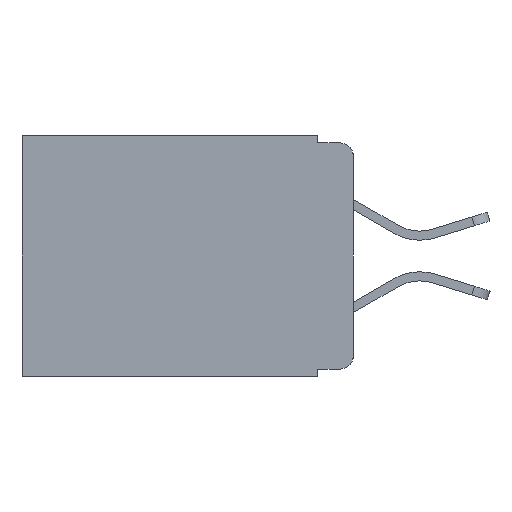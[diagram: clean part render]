
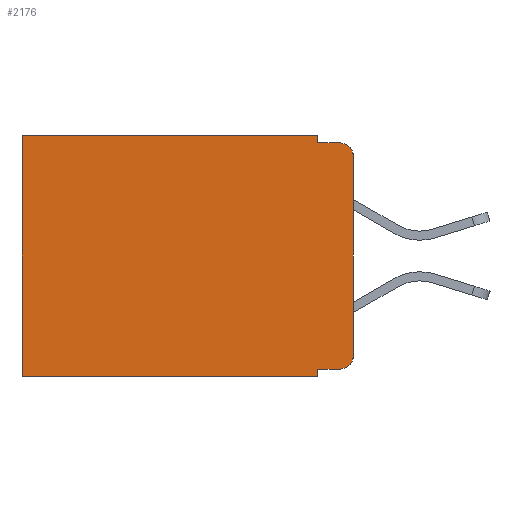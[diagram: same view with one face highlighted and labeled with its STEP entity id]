
A CAD part, left-side view. The second image highlights one B-rep face of the part: STEP entity #2176.
In plain terms, the highlighted planar face has unit normal (-1, 0, 0).
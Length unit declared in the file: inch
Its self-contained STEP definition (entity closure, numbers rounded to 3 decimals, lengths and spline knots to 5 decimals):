
#89 = DIRECTION ( 'NONE',  ( 0., 0., -1. ) ) ;
#152 = CARTESIAN_POINT ( 'NONE',  ( 0.298, 0., -0.313 ) ) ;
#309 = ORIENTED_EDGE ( 'NONE', *, *, #8397, .T. ) ;
#338 = DIRECTION ( 'NONE',  ( 0., 1., 0. ) ) ;
#526 = DIRECTION ( 'NONE',  ( 0., -1., 0. ) ) ;
#675 = VECTOR ( 'NONE', #7636, 39.37008 ) ;
#694 = CIRCLE ( 'NONE', #1011, 0.02 ) ;
#705 = CIRCLE ( 'NONE', #3646, 0.02 ) ;
#892 = ORIENTED_EDGE ( 'NONE', *, *, #9301, .F. ) ;
#983 = CARTESIAN_POINT ( 'NONE',  ( 0.298, 0., 0. ) ) ;
#1011 = AXIS2_PLACEMENT_3D ( 'NONE', #6147, #4822, #6840 ) ;
#1178 = ORIENTED_EDGE ( 'NONE', *, *, #4359, .T. ) ;
#1251 = CARTESIAN_POINT ( 'NONE',  ( 0.298, 0.051, -0.333 ) ) ;
#1271 = VECTOR ( 'NONE', #1478, 39.37008 ) ;
#1478 = DIRECTION ( 'NONE',  ( 0., 1., 0. ) ) ;
#1589 = VERTEX_POINT ( 'NONE', #152 ) ;
#1775 = EDGE_CURVE ( 'NONE', #8968, #4021, #9568, .T. ) ;
#1894 = DIRECTION ( 'NONE',  ( 0., 0., -1. ) ) ;
#1939 = EDGE_CURVE ( 'NONE', #4628, #1589, #705, .T. ) ;
#1988 = PLANE ( 'NONE',  #2154 ) ;
#2154 = AXIS2_PLACEMENT_3D ( 'NONE', #3387, #4264, #2862 ) ;
#2176 = ADVANCED_FACE ( 'NONE', ( #7290 ), #1988, .F. ) ;
#2305 = VERTEX_POINT ( 'NONE', #9011 ) ;
#2339 = VERTEX_POINT ( 'NONE', #7537 ) ;
#2573 = EDGE_LOOP ( 'NONE', ( #6228, #1178, #892, #5201, #9471, #3270, #3724, #5492, #309, #3844 ) ) ;
#2699 = CARTESIAN_POINT ( 'NONE',  ( 0.298, 0.473, 0. ) ) ;
#2757 = LINE ( 'NONE', #8126, #1271 ) ;
#2845 = CARTESIAN_POINT ( 'NONE',  ( 0.298, 0.051, 0. ) ) ;
#2862 = DIRECTION ( 'NONE',  ( 0., 0., -1. ) ) ;
#3270 = ORIENTED_EDGE ( 'NONE', *, *, #4654, .T. ) ;
#3387 = CARTESIAN_POINT ( 'NONE',  ( 0.298, 0., 0. ) ) ;
#3646 = AXIS2_PLACEMENT_3D ( 'NONE', #6661, #6813, #5195 ) ;
#3724 = ORIENTED_EDGE ( 'NONE', *, *, #7946, .F. ) ;
#3821 = EDGE_CURVE ( 'NONE', #2339, #1589, #9248, .T. ) ;
#3844 = ORIENTED_EDGE ( 'NONE', *, *, #1939, .T. ) ;
#3999 = CARTESIAN_POINT ( 'NONE',  ( 0.298, 0., 0. ) ) ;
#4021 = VERTEX_POINT ( 'NONE', #5648 ) ;
#4184 = VECTOR ( 'NONE', #6617, 39.37008 ) ;
#4264 = DIRECTION ( 'NONE',  ( 1., 0., 0. ) ) ;
#4359 = EDGE_CURVE ( 'NONE', #2339, #5888, #694, .T. ) ;
#4366 = VECTOR ( 'NONE', #1894, 39.37008 ) ;
#4402 = CARTESIAN_POINT ( 'NONE',  ( 0.298, 0.473, 0. ) ) ;
#4628 = VERTEX_POINT ( 'NONE', #6039 ) ;
#4654 = EDGE_CURVE ( 'NONE', #5810, #9286, #8153, .T. ) ;
#4675 = CARTESIAN_POINT ( 'NONE',  ( 0.298, 0.051, 0. ) ) ;
#4822 = DIRECTION ( 'NONE',  ( -1., 0., 0. ) ) ;
#4914 = LINE ( 'NONE', #1251, #9352 ) ;
#5195 = DIRECTION ( 'NONE',  ( 0., 0., -1. ) ) ;
#5201 = ORIENTED_EDGE ( 'NONE', *, *, #1775, .F. ) ;
#5300 = VERTEX_POINT ( 'NONE', #9343 ) ;
#5492 = ORIENTED_EDGE ( 'NONE', *, *, #7673, .F. ) ;
#5648 = CARTESIAN_POINT ( 'NONE',  ( 0.298, 0.051, -0.01 ) ) ;
#5810 = VERTEX_POINT ( 'NONE', #2699 ) ;
#5888 = VERTEX_POINT ( 'NONE', #8154 ) ;
#6039 = CARTESIAN_POINT ( 'NONE',  ( 0.298, 0.02, -0.333 ) ) ;
#6076 = VECTOR ( 'NONE', #338, 39.37008 ) ;
#6147 = CARTESIAN_POINT ( 'NONE',  ( 0.298, 0.02, -0.03 ) ) ;
#6175 = VECTOR ( 'NONE', #89, 39.37008 ) ;
#6228 = ORIENTED_EDGE ( 'NONE', *, *, #3821, .F. ) ;
#6571 = CARTESIAN_POINT ( 'NONE',  ( 0.298, 0.051, -0.01 ) ) ;
#6617 = DIRECTION ( 'NONE',  ( 0., -1., 0. ) ) ;
#6661 = CARTESIAN_POINT ( 'NONE',  ( 0.298, 0.02, -0.313 ) ) ;
#6813 = DIRECTION ( 'NONE',  ( -1., 0., 0. ) ) ;
#6840 = DIRECTION ( 'NONE',  ( 0., 0., -1. ) ) ;
#6943 = LINE ( 'NONE', #3999, #6076 ) ;
#7290 = FACE_OUTER_BOUND ( 'NONE', #2573, .T. ) ;
#7452 = LINE ( 'NONE', #6571, #4184 ) ;
#7537 = CARTESIAN_POINT ( 'NONE',  ( 0.298, 0., -0.03 ) ) ;
#7636 = DIRECTION ( 'NONE',  ( 0., 0., -1. ) ) ;
#7673 = EDGE_CURVE ( 'NONE', #5300, #2305, #7873, .T. ) ;
#7873 = LINE ( 'NONE', #9338, #4366 ) ;
#7946 = EDGE_CURVE ( 'NONE', #2305, #9286, #2757, .T. ) ;
#8126 = CARTESIAN_POINT ( 'NONE',  ( 0.298, 0., -0.343 ) ) ;
#8139 = EDGE_CURVE ( 'NONE', #8968, #5810, #6943, .T. ) ;
#8153 = LINE ( 'NONE', #4402, #6175 ) ;
#8154 = CARTESIAN_POINT ( 'NONE',  ( 0.298, 0.02, -0.01 ) ) ;
#8283 = CARTESIAN_POINT ( 'NONE',  ( 0.298, 0.473, -0.343 ) ) ;
#8397 = EDGE_CURVE ( 'NONE', #5300, #4628, #4914, .T. ) ;
#8800 = VECTOR ( 'NONE', #8902, 39.37008 ) ;
#8902 = DIRECTION ( 'NONE',  ( 0., 0., -1. ) ) ;
#8968 = VERTEX_POINT ( 'NONE', #4675 ) ;
#9011 = CARTESIAN_POINT ( 'NONE',  ( 0.298, 0.051, -0.343 ) ) ;
#9248 = LINE ( 'NONE', #983, #675 ) ;
#9286 = VERTEX_POINT ( 'NONE', #8283 ) ;
#9301 = EDGE_CURVE ( 'NONE', #4021, #5888, #7452, .T. ) ;
#9338 = CARTESIAN_POINT ( 'NONE',  ( 0.298, 0.051, 0. ) ) ;
#9343 = CARTESIAN_POINT ( 'NONE',  ( 0.298, 0.051, -0.333 ) ) ;
#9352 = VECTOR ( 'NONE', #526, 39.37008 ) ;
#9471 = ORIENTED_EDGE ( 'NONE', *, *, #8139, .T. ) ;
#9568 = LINE ( 'NONE', #2845, #8800 ) ;
